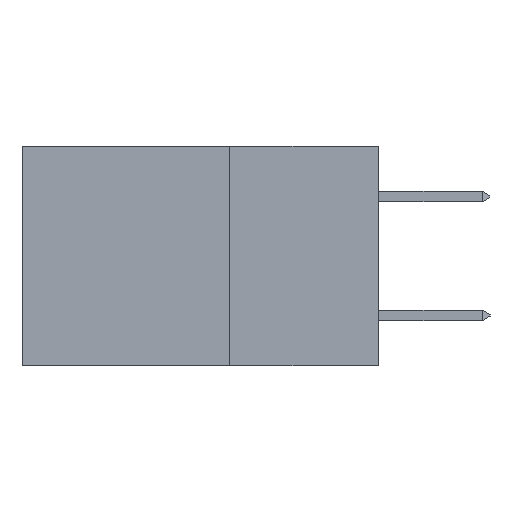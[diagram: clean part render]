
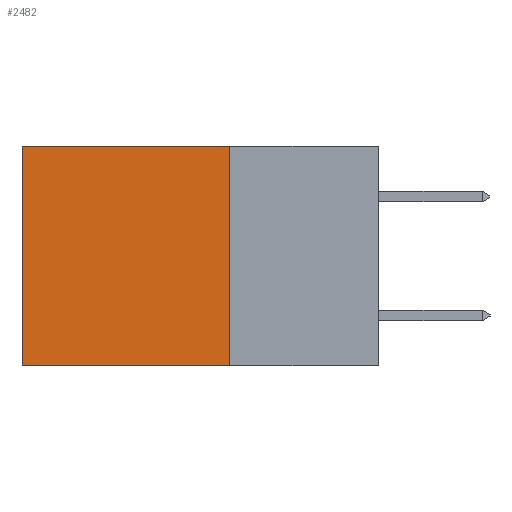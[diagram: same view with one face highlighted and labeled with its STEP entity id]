
A CAD part, left-side view. The second image highlights one B-rep face of the part: STEP entity #2482.
In plain terms, the highlighted planar face has unit normal (-1, 0, 0).
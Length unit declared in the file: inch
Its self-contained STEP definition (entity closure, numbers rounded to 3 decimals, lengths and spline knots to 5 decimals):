
#553 = VECTOR ( 'NONE', #11146, 39.37008 ) ;
#1450 = VERTEX_POINT ( 'NONE', #11132 ) ;
#1871 = EDGE_CURVE ( 'NONE', #9867, #2076, #11262, .T. ) ;
#2041 = LINE ( 'NONE', #5852, #13098 ) ;
#2076 = VERTEX_POINT ( 'NONE', #4389 ) ;
#2279 = DIRECTION ( 'NONE',  ( 0., 0., -1. ) ) ;
#2482 = ADVANCED_FACE ( 'NONE', ( #4510 ), #6160, .F. ) ;
#2747 = CARTESIAN_POINT ( 'NONE',  ( 0.2615, 0.25, -0.37 ) ) ;
#3523 = VERTEX_POINT ( 'NONE', #6260 ) ;
#4389 = CARTESIAN_POINT ( 'NONE',  ( 0.2615, 0.25, -0.37 ) ) ;
#4510 = FACE_OUTER_BOUND ( 'NONE', #9167, .T. ) ;
#4959 = CARTESIAN_POINT ( 'NONE',  ( 0.2615, 0.25, 0. ) ) ;
#5329 = DIRECTION ( 'NONE',  ( 0., 0., -1. ) ) ;
#5393 = DIRECTION ( 'NONE',  ( 1., 0., 0. ) ) ;
#5531 = AXIS2_PLACEMENT_3D ( 'NONE', #5572, #5393, #5329 ) ;
#5572 = CARTESIAN_POINT ( 'NONE',  ( 0.2615, 0.25, -0.37 ) ) ;
#5575 = VECTOR ( 'NONE', #2279, 39.37008 ) ;
#5852 = CARTESIAN_POINT ( 'NONE',  ( 0.2615, 0.6, -0.37 ) ) ;
#6155 = ORIENTED_EDGE ( 'NONE', *, *, #8801, .F. ) ;
#6160 = PLANE ( 'NONE',  #5531 ) ;
#6212 = DIRECTION ( 'NONE',  ( 0., 0., -1. ) ) ;
#6260 = CARTESIAN_POINT ( 'NONE',  ( 0.2615, 0.6, -0.37 ) ) ;
#6703 = EDGE_CURVE ( 'NONE', #9867, #1450, #11453, .T. ) ;
#8079 = ORIENTED_EDGE ( 'NONE', *, *, #1871, .F. ) ;
#8766 = ORIENTED_EDGE ( 'NONE', *, *, #6703, .T. ) ;
#8801 = EDGE_CURVE ( 'NONE', #2076, #3523, #11748, .T. ) ;
#9167 = EDGE_LOOP ( 'NONE', ( #13108, #6155, #8079, #8766 ) ) ;
#9835 = EDGE_CURVE ( 'NONE', #1450, #3523, #2041, .T. ) ;
#9867 = VERTEX_POINT ( 'NONE', #4959 ) ;
#11132 = CARTESIAN_POINT ( 'NONE',  ( 0.2615, 0.6, 0. ) ) ;
#11140 = VECTOR ( 'NONE', #11433, 39.37008 ) ;
#11146 = DIRECTION ( 'NONE',  ( 0., 1., 0. ) ) ;
#11262 = LINE ( 'NONE', #2747, #5575 ) ;
#11433 = DIRECTION ( 'NONE',  ( 0., 1., 0. ) ) ;
#11453 = LINE ( 'NONE', #11577, #11140 ) ;
#11577 = CARTESIAN_POINT ( 'NONE',  ( 0.2615, 0.25, 0. ) ) ;
#11684 = CARTESIAN_POINT ( 'NONE',  ( 0.2615, 0.25, -0.37 ) ) ;
#11748 = LINE ( 'NONE', #11684, #553 ) ;
#13098 = VECTOR ( 'NONE', #6212, 39.37008 ) ;
#13108 = ORIENTED_EDGE ( 'NONE', *, *, #9835, .T. ) ;
